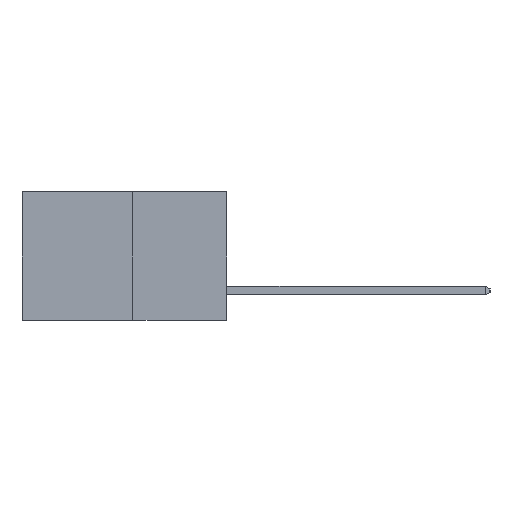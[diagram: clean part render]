
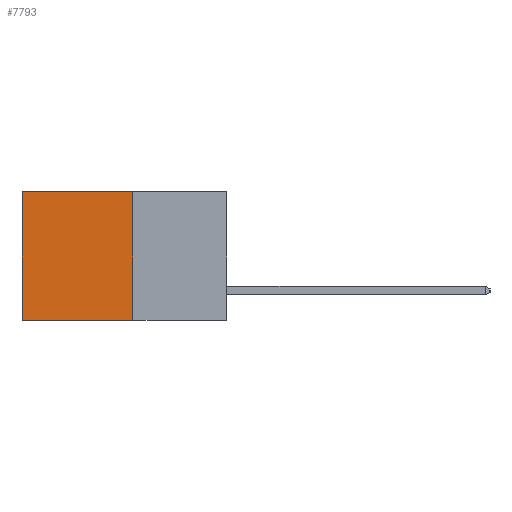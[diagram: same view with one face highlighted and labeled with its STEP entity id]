
A CAD part, left-side view. The second image highlights one B-rep face of the part: STEP entity #7793.
In plain terms, the highlighted planar face has unit normal (-1, 0, 0).
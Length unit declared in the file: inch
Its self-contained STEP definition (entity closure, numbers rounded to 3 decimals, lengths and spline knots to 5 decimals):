
#358 = VERTEX_POINT ( 'NONE', #9255 ) ;
#812 = EDGE_CURVE ( 'NONE', #358, #8026, #9275, .T. ) ;
#1006 = AXIS2_PLACEMENT_3D ( 'NONE', #4141, #3816, #3729 ) ;
#1600 = EDGE_CURVE ( 'NONE', #8026, #11662, #13535, .T. ) ;
#2224 = ORIENTED_EDGE ( 'NONE', *, *, #8589, .T. ) ;
#2282 = ORIENTED_EDGE ( 'NONE', *, *, #1600, .F. ) ;
#2300 = ORIENTED_EDGE ( 'NONE', *, *, #812, .F. ) ;
#2336 = ORIENTED_EDGE ( 'NONE', *, *, #12670, .T. ) ;
#2340 = VECTOR ( 'NONE', #6951, 39.37008 ) ;
#2567 = FACE_OUTER_BOUND ( 'NONE', #7796, .T. ) ;
#3129 = CARTESIAN_POINT ( 'NONE',  ( 0.277, 0.59, -0.37 ) ) ;
#3729 = DIRECTION ( 'NONE',  ( 0., 0., -1. ) ) ;
#3816 = DIRECTION ( 'NONE',  ( 1., 0., 0. ) ) ;
#4079 = PLANE ( 'NONE',  #1006 ) ;
#4141 = CARTESIAN_POINT ( 'NONE',  ( 0.277, 0.27, -0.37 ) ) ;
#4988 = DIRECTION ( 'NONE',  ( 0., 0., -1. ) ) ;
#5053 = CARTESIAN_POINT ( 'NONE',  ( 0.277, 0.59, -0.37 ) ) ;
#5142 = VECTOR ( 'NONE', #9856, 39.37008 ) ;
#5534 = LINE ( 'NONE', #6411, #2340 ) ;
#6404 = VECTOR ( 'NONE', #9470, 39.37008 ) ;
#6411 = CARTESIAN_POINT ( 'NONE',  ( 0.277, 0.27, 0. ) ) ;
#6951 = DIRECTION ( 'NONE',  ( 0., 1., 0. ) ) ;
#7793 = ADVANCED_FACE ( 'NONE', ( #2567 ), #4079, .F. ) ;
#7796 = EDGE_LOOP ( 'NONE', ( #2224, #2282, #2300, #2336 ) ) ;
#8026 = VERTEX_POINT ( 'NONE', #11809 ) ;
#8589 = EDGE_CURVE ( 'NONE', #13069, #11662, #9975, .T. ) ;
#9255 = CARTESIAN_POINT ( 'NONE',  ( 0.277, 0.27, 0. ) ) ;
#9275 = LINE ( 'NONE', #11839, #6404 ) ;
#9470 = DIRECTION ( 'NONE',  ( 0., 0., -1. ) ) ;
#9856 = DIRECTION ( 'NONE',  ( 0., 1., 0. ) ) ;
#9975 = LINE ( 'NONE', #5053, #12024 ) ;
#10452 = CARTESIAN_POINT ( 'NONE',  ( 0.277, 0.27, -0.37 ) ) ;
#11662 = VERTEX_POINT ( 'NONE', #3129 ) ;
#11809 = CARTESIAN_POINT ( 'NONE',  ( 0.277, 0.27, -0.37 ) ) ;
#11839 = CARTESIAN_POINT ( 'NONE',  ( 0.277, 0.27, -0.37 ) ) ;
#12024 = VECTOR ( 'NONE', #4988, 39.37008 ) ;
#12574 = CARTESIAN_POINT ( 'NONE',  ( 0.277, 0.59, 0. ) ) ;
#12670 = EDGE_CURVE ( 'NONE', #358, #13069, #5534, .T. ) ;
#13069 = VERTEX_POINT ( 'NONE', #12574 ) ;
#13535 = LINE ( 'NONE', #10452, #5142 ) ;
